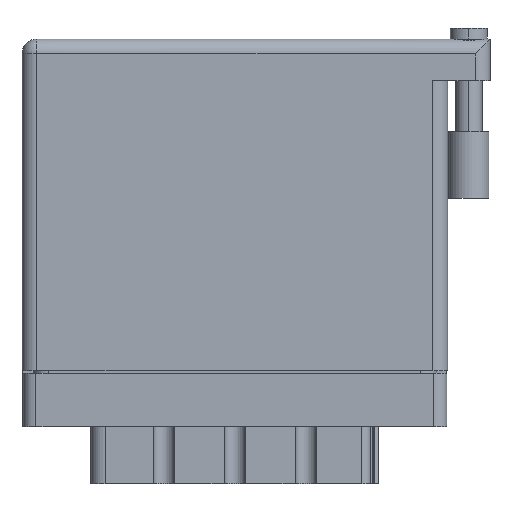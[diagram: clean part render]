
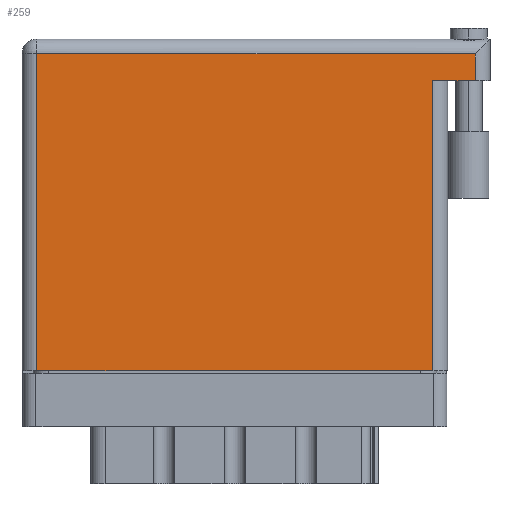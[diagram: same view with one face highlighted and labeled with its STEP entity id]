
A CAD part, front view. The second image highlights one B-rep face of the part: STEP entity #259.
In plain terms, the highlighted face is planar.
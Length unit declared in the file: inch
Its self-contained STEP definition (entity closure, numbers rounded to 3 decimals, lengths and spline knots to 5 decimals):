
#119 = ORIENTED_EDGE ( 'NONE', *, *, #20813, .T. ) ;
#259 = ADVANCED_FACE ( 'NONE', ( #24325 ), #24840, .F. ) ;
#344 = LINE ( 'NONE', #25978, #7542 ) ;
#1578 = CARTESIAN_POINT ( 'NONE',  ( 0., 1.566, 0. ) ) ;
#2030 = CARTESIAN_POINT ( 'NONE',  ( 0., 1.496, 0. ) ) ;
#2054 = DIRECTION ( 'NONE',  ( 1., 0., 0. ) ) ;
#2516 = DIRECTION ( 'NONE',  ( -1., 0., 0. ) ) ;
#2971 = VECTOR ( 'NONE', #2054, 39.37008 ) ;
#4559 = DIRECTION ( 'NONE',  ( -1., 0., 0. ) ) ;
#4939 = LINE ( 'NONE', #2030, #11642 ) ;
#6200 = LINE ( 'NONE', #32530, #14735 ) ;
#6675 = CARTESIAN_POINT ( 'NONE',  ( 0.07, 0., 0. ) ) ;
#7074 = DIRECTION ( 'NONE',  ( 0., 1., 0. ) ) ;
#7542 = VECTOR ( 'NONE', #23398, 39.37008 ) ;
#8717 = EDGE_CURVE ( 'NONE', #29565, #22484, #4939, .T. ) ;
#9956 = CARTESIAN_POINT ( 'NONE',  ( 2.208, 1.369, 0. ) ) ;
#10467 = DIRECTION ( 'NONE',  ( -1., 0., 0. ) ) ;
#10579 = DIRECTION ( 'NONE',  ( 0., 0., -1. ) ) ;
#11509 = EDGE_CURVE ( 'NONE', #22484, #35250, #11779, .T. ) ;
#11642 = VECTOR ( 'NONE', #2516, 39.37008 ) ;
#11779 = LINE ( 'NONE', #15557, #16644 ) ;
#12019 = ORIENTED_EDGE ( 'NONE', *, *, #11509, .T. ) ;
#12043 = EDGE_CURVE ( 'NONE', #15069, #35133, #32973, .T. ) ;
#12866 = CARTESIAN_POINT ( 'NONE',  ( 2.138, 1.496, 0. ) ) ;
#13382 = EDGE_CURVE ( 'NONE', #32536, #35133, #344, .T. ) ;
#13390 = ORIENTED_EDGE ( 'NONE', *, *, #32663, .T. ) ;
#13921 = ORIENTED_EDGE ( 'NONE', *, *, #8717, .T. ) ;
#14735 = VECTOR ( 'NONE', #7074, 39.37008 ) ;
#15069 = VERTEX_POINT ( 'NONE', #20617 ) ;
#15557 = CARTESIAN_POINT ( 'NONE',  ( 0.07, 0., 0. ) ) ;
#16644 = VECTOR ( 'NONE', #26833, 39.37008 ) ;
#17634 = CARTESIAN_POINT ( 'NONE',  ( 1.938, 1.369, 0. ) ) ;
#19897 = ORIENTED_EDGE ( 'NONE', *, *, #12043, .F. ) ;
#20617 = CARTESIAN_POINT ( 'NONE',  ( 2.138, 1.369, 0. ) ) ;
#20734 = CARTESIAN_POINT ( 'NONE',  ( 0.07, 1.496, 0. ) ) ;
#20813 = EDGE_CURVE ( 'NONE', #15069, #29565, #6200, .T. ) ;
#22484 = VERTEX_POINT ( 'NONE', #20734 ) ;
#23398 = DIRECTION ( 'NONE',  ( 0., 1., 0. ) ) ;
#24325 = FACE_OUTER_BOUND ( 'NONE', #34654, .T. ) ;
#24840 = PLANE ( 'NONE',  #24927 ) ;
#24927 = AXIS2_PLACEMENT_3D ( 'NONE', #1578, #10579, #10467 ) ;
#25399 = VECTOR ( 'NONE', #4559, 39.37008 ) ;
#25978 = CARTESIAN_POINT ( 'NONE',  ( 1.938, 1.369, 0. ) ) ;
#26833 = DIRECTION ( 'NONE',  ( 0., -1., 0. ) ) ;
#27312 = CARTESIAN_POINT ( 'NONE',  ( 1.938, 0., 0. ) ) ;
#29565 = VERTEX_POINT ( 'NONE', #12866 ) ;
#29671 = LINE ( 'NONE', #35990, #2971 ) ;
#32530 = CARTESIAN_POINT ( 'NONE',  ( 2.138, 1.566, 0. ) ) ;
#32536 = VERTEX_POINT ( 'NONE', #27312 ) ;
#32663 = EDGE_CURVE ( 'NONE', #35250, #32536, #29671, .T. ) ;
#32973 = LINE ( 'NONE', #9956, #25399 ) ;
#34427 = ORIENTED_EDGE ( 'NONE', *, *, #13382, .T. ) ;
#34654 = EDGE_LOOP ( 'NONE', ( #13390, #34427, #19897, #119, #13921, #12019 ) ) ;
#35133 = VERTEX_POINT ( 'NONE', #17634 ) ;
#35250 = VERTEX_POINT ( 'NONE', #6675 ) ;
#35990 = CARTESIAN_POINT ( 'NONE',  ( 0., 0., 0. ) ) ;
